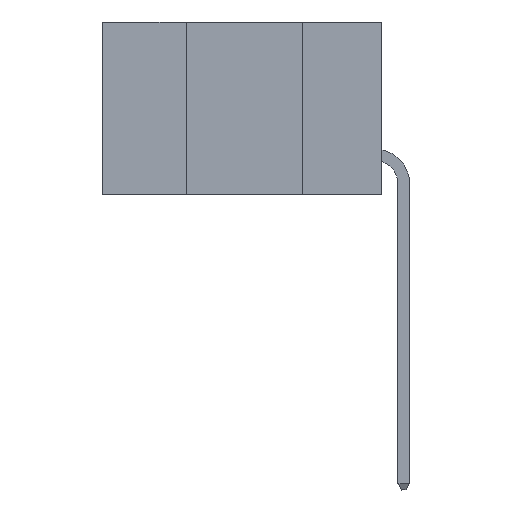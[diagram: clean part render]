
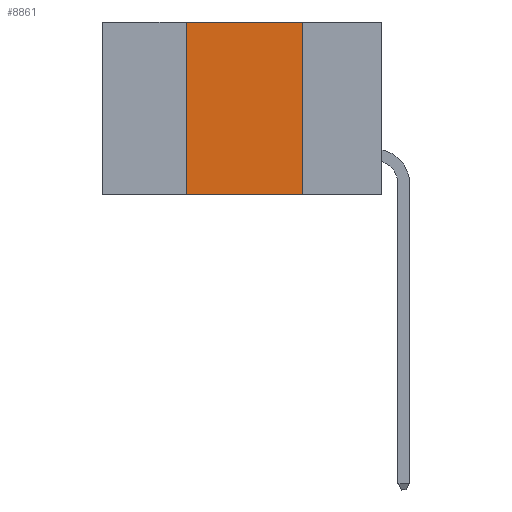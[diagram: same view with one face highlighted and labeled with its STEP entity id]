
A CAD part, left-side view. The second image highlights one B-rep face of the part: STEP entity #8861.
In plain terms, the highlighted planar face has unit normal (-1, 0, 0).
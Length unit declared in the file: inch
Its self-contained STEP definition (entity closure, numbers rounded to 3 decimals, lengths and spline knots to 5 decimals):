
#1459 = DIRECTION ( 'NONE',  ( 0., -1., 0. ) ) ;
#1857 = EDGE_CURVE ( 'NONE', #28747, #19614, #22927, .T. ) ;
#5633 = ORIENTED_EDGE ( 'NONE', *, *, #35812, .F. ) ;
#6093 = EDGE_CURVE ( 'NONE', #9805, #23067, #7552, .T. ) ;
#7552 = LINE ( 'NONE', #32520, #23403 ) ;
#8186 = DIRECTION ( 'NONE',  ( 0., -1., 0. ) ) ;
#8861 = ADVANCED_FACE ( 'NONE', ( #35559 ), #13082, .F. ) ;
#9805 = VERTEX_POINT ( 'NONE', #37537 ) ;
#9991 = CARTESIAN_POINT ( 'NONE',  ( 0., 0.17, -0.37 ) ) ;
#10340 = EDGE_CURVE ( 'NONE', #9805, #28747, #40511, .T. ) ;
#13082 = PLANE ( 'NONE',  #40107 ) ;
#13430 = EDGE_LOOP ( 'NONE', ( #5633, #34077, #24945, #37551 ) ) ;
#15479 = LINE ( 'NONE', #34934, #33763 ) ;
#17735 = CARTESIAN_POINT ( 'NONE',  ( 0., 0.6, 0. ) ) ;
#18247 = DIRECTION ( 'NONE',  ( 0., 0., 1. ) ) ;
#19614 = VERTEX_POINT ( 'NONE', #24088 ) ;
#20125 = DIRECTION ( 'NONE',  ( 1., 0., 0. ) ) ;
#20995 = VECTOR ( 'NONE', #8186, 39.37008 ) ;
#22640 = CARTESIAN_POINT ( 'NONE',  ( 0., 0.6, 0. ) ) ;
#22645 = VECTOR ( 'NONE', #18247, 39.37008 ) ;
#22730 = CARTESIAN_POINT ( 'NONE',  ( 0., 0.42, 0. ) ) ;
#22927 = LINE ( 'NONE', #17735, #20995 ) ;
#23067 = VERTEX_POINT ( 'NONE', #9991 ) ;
#23403 = VECTOR ( 'NONE', #1459, 39.37008 ) ;
#24088 = CARTESIAN_POINT ( 'NONE',  ( 0., 0.17, 0. ) ) ;
#24327 = CARTESIAN_POINT ( 'NONE',  ( 0., 0.42, 0. ) ) ;
#24945 = ORIENTED_EDGE ( 'NONE', *, *, #10340, .F. ) ;
#28747 = VERTEX_POINT ( 'NONE', #22730 ) ;
#28786 = DIRECTION ( 'NONE',  ( 0., 0., -1. ) ) ;
#32520 = CARTESIAN_POINT ( 'NONE',  ( 0., 0.6, -0.37 ) ) ;
#33763 = VECTOR ( 'NONE', #28786, 39.37008 ) ;
#33802 = DIRECTION ( 'NONE',  ( 0., 0., -1. ) ) ;
#34077 = ORIENTED_EDGE ( 'NONE', *, *, #1857, .F. ) ;
#34934 = CARTESIAN_POINT ( 'NONE',  ( 0., 0.17, 0. ) ) ;
#35559 = FACE_OUTER_BOUND ( 'NONE', #13430, .T. ) ;
#35812 = EDGE_CURVE ( 'NONE', #19614, #23067, #15479, .T. ) ;
#37537 = CARTESIAN_POINT ( 'NONE',  ( 0., 0.42, -0.37 ) ) ;
#37551 = ORIENTED_EDGE ( 'NONE', *, *, #6093, .T. ) ;
#40107 = AXIS2_PLACEMENT_3D ( 'NONE', #22640, #20125, #33802 ) ;
#40511 = LINE ( 'NONE', #24327, #22645 ) ;
